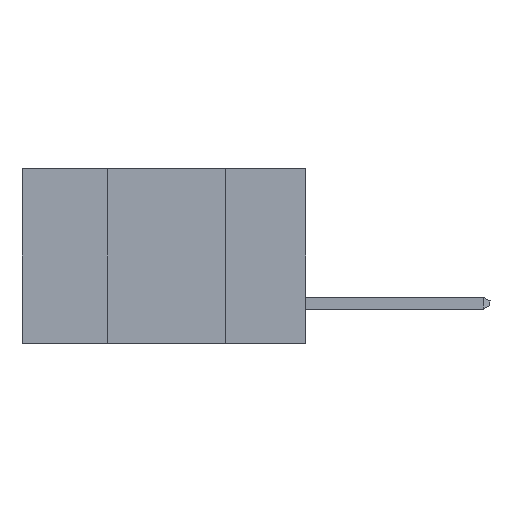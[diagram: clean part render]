
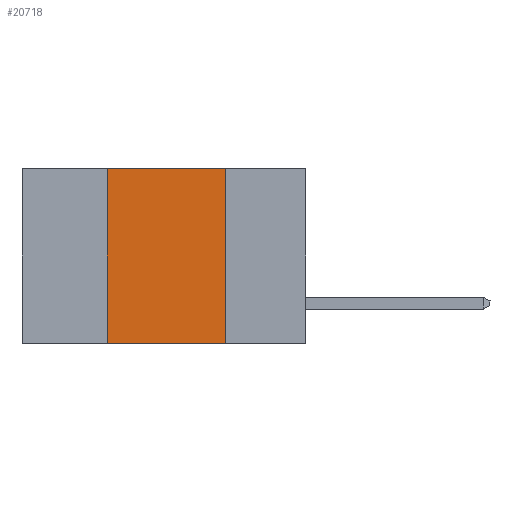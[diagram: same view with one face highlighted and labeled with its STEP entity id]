
A CAD part, left-side view. The second image highlights one B-rep face of the part: STEP entity #20718.
In plain terms, the highlighted planar face has unit normal (-1, 0, 0).
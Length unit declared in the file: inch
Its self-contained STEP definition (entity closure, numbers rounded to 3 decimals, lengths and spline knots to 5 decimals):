
#351 = DIRECTION ( 'NONE',  ( 1., 0., 0. ) ) ;
#669 = VECTOR ( 'NONE', #15843, 39.37008 ) ;
#1725 = CARTESIAN_POINT ( 'NONE',  ( 0., 0.42, 0. ) ) ;
#1938 = VECTOR ( 'NONE', #9284, 39.37008 ) ;
#1963 = EDGE_LOOP ( 'NONE', ( #15493, #5706, #10925, #5666 ) ) ;
#2045 = EDGE_CURVE ( 'NONE', #17697, #3443, #16708, .T. ) ;
#2515 = EDGE_CURVE ( 'NONE', #3179, #17697, #23018, .T. ) ;
#3179 = VERTEX_POINT ( 'NONE', #1725 ) ;
#3443 = VERTEX_POINT ( 'NONE', #17626 ) ;
#3757 = FACE_OUTER_BOUND ( 'NONE', #1963, .T. ) ;
#3855 = CARTESIAN_POINT ( 'NONE',  ( 0., 0.17, -0.37 ) ) ;
#4673 = LINE ( 'NONE', #11897, #669 ) ;
#5170 = DIRECTION ( 'NONE',  ( 0., 0., 1. ) ) ;
#5666 = ORIENTED_EDGE ( 'NONE', *, *, #19867, .T. ) ;
#5706 = ORIENTED_EDGE ( 'NONE', *, *, #2515, .F. ) ;
#5861 = VERTEX_POINT ( 'NONE', #19495 ) ;
#7433 = DIRECTION ( 'NONE',  ( 0., 0., -1. ) ) ;
#9284 = DIRECTION ( 'NONE',  ( 0., 0., -1. ) ) ;
#10290 = VECTOR ( 'NONE', #13827, 39.37008 ) ;
#10925 = ORIENTED_EDGE ( 'NONE', *, *, #19733, .F. ) ;
#11209 = AXIS2_PLACEMENT_3D ( 'NONE', #16493, #351, #7433 ) ;
#11897 = CARTESIAN_POINT ( 'NONE',  ( 0., 0.6, -0.37 ) ) ;
#12716 = CARTESIAN_POINT ( 'NONE',  ( 0., 0.42, -0.37 ) ) ;
#13240 = CARTESIAN_POINT ( 'NONE',  ( 0., 0.17, 0. ) ) ;
#13485 = VECTOR ( 'NONE', #5170, 39.37008 ) ;
#13827 = DIRECTION ( 'NONE',  ( 0., -1., 0. ) ) ;
#14417 = PLANE ( 'NONE',  #11209 ) ;
#15493 = ORIENTED_EDGE ( 'NONE', *, *, #2045, .F. ) ;
#15843 = DIRECTION ( 'NONE',  ( 0., -1., 0. ) ) ;
#16493 = CARTESIAN_POINT ( 'NONE',  ( 0., 0.6, 0. ) ) ;
#16708 = LINE ( 'NONE', #3855, #1938 ) ;
#17626 = CARTESIAN_POINT ( 'NONE',  ( 0., 0.17, -0.37 ) ) ;
#17697 = VERTEX_POINT ( 'NONE', #13240 ) ;
#19438 = CARTESIAN_POINT ( 'NONE',  ( 0., 0.6, 0. ) ) ;
#19495 = CARTESIAN_POINT ( 'NONE',  ( 0., 0.42, -0.37 ) ) ;
#19733 = EDGE_CURVE ( 'NONE', #5861, #3179, #21795, .T. ) ;
#19867 = EDGE_CURVE ( 'NONE', #5861, #3443, #4673, .T. ) ;
#20718 = ADVANCED_FACE ( 'NONE', ( #3757 ), #14417, .F. ) ;
#21795 = LINE ( 'NONE', #12716, #13485 ) ;
#23018 = LINE ( 'NONE', #19438, #10290 ) ;
